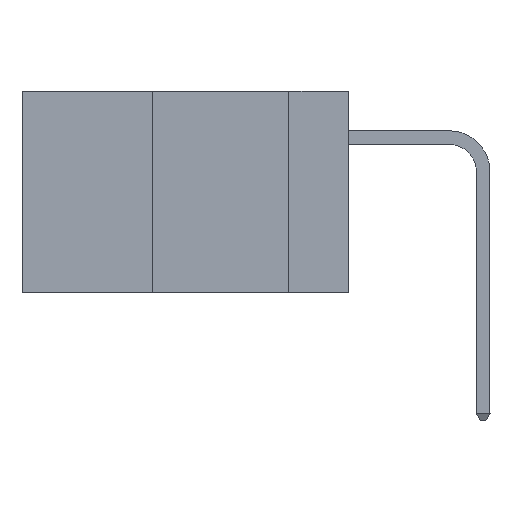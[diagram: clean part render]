
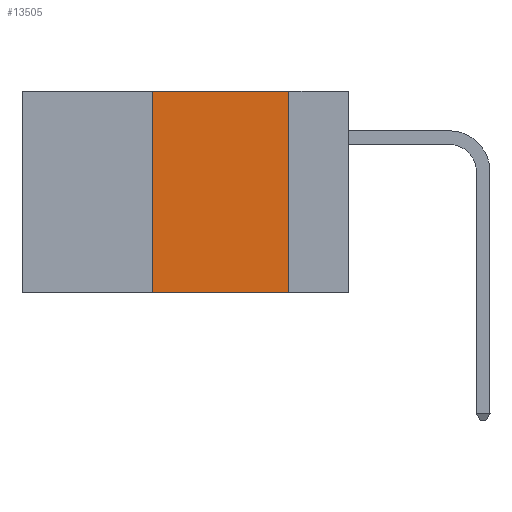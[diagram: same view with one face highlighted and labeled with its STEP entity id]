
A CAD part, left-side view. The second image highlights one B-rep face of the part: STEP entity #13505.
In plain terms, the highlighted planar face has unit normal (-1, 0, 0).
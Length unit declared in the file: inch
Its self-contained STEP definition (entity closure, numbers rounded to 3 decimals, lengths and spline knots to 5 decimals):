
#1385 = EDGE_CURVE ( 'NONE', #3851, #40152, #15248, .T. ) ;
#3851 = VERTEX_POINT ( 'NONE', #22185 ) ;
#4077 = CARTESIAN_POINT ( 'NONE',  ( 0., 0.36, 0. ) ) ;
#4573 = DIRECTION ( 'NONE',  ( 0., 0., -1. ) ) ;
#5315 = CARTESIAN_POINT ( 'NONE',  ( 0., 0.11, 0. ) ) ;
#6970 = VECTOR ( 'NONE', #32015, 39.37008 ) ;
#7897 = CARTESIAN_POINT ( 'NONE',  ( 0., 0.36, 0. ) ) ;
#8837 = CARTESIAN_POINT ( 'NONE',  ( 0., 0.6, 0. ) ) ;
#9611 = LINE ( 'NONE', #26953, #22558 ) ;
#10759 = ORIENTED_EDGE ( 'NONE', *, *, #25323, .T. ) ;
#11926 = EDGE_CURVE ( 'NONE', #40152, #25382, #15953, .T. ) ;
#12947 = DIRECTION ( 'NONE',  ( 0., -1., 0. ) ) ;
#13505 = ADVANCED_FACE ( 'NONE', ( #25249 ), #34825, .F. ) ;
#15248 = LINE ( 'NONE', #7897, #15716 ) ;
#15716 = VECTOR ( 'NONE', #28805, 39.37008 ) ;
#15953 = LINE ( 'NONE', #8837, #27984 ) ;
#17704 = DIRECTION ( 'NONE',  ( 1., 0., 0. ) ) ;
#22185 = CARTESIAN_POINT ( 'NONE',  ( 0., 0.36, -0.37 ) ) ;
#22558 = VECTOR ( 'NONE', #12947, 39.37008 ) ;
#23162 = EDGE_LOOP ( 'NONE', ( #31572, #28137, #36270, #10759 ) ) ;
#25249 = FACE_OUTER_BOUND ( 'NONE', #23162, .T. ) ;
#25323 = EDGE_CURVE ( 'NONE', #3851, #27844, #9611, .T. ) ;
#25382 = VERTEX_POINT ( 'NONE', #40768 ) ;
#26953 = CARTESIAN_POINT ( 'NONE',  ( 0., 0.6, -0.37 ) ) ;
#27844 = VERTEX_POINT ( 'NONE', #35292 ) ;
#27984 = VECTOR ( 'NONE', #39996, 39.37008 ) ;
#28137 = ORIENTED_EDGE ( 'NONE', *, *, #11926, .F. ) ;
#28805 = DIRECTION ( 'NONE',  ( 0., 0., 1. ) ) ;
#31572 = ORIENTED_EDGE ( 'NONE', *, *, #38902, .F. ) ;
#31579 = LINE ( 'NONE', #5315, #6970 ) ;
#31980 = AXIS2_PLACEMENT_3D ( 'NONE', #35272, #17704, #4573 ) ;
#32015 = DIRECTION ( 'NONE',  ( 0., 0., -1. ) ) ;
#34825 = PLANE ( 'NONE',  #31980 ) ;
#35272 = CARTESIAN_POINT ( 'NONE',  ( 0., 0.6, 0. ) ) ;
#35292 = CARTESIAN_POINT ( 'NONE',  ( 0., 0.11, -0.37 ) ) ;
#36270 = ORIENTED_EDGE ( 'NONE', *, *, #1385, .F. ) ;
#38902 = EDGE_CURVE ( 'NONE', #25382, #27844, #31579, .T. ) ;
#39996 = DIRECTION ( 'NONE',  ( 0., -1., 0. ) ) ;
#40152 = VERTEX_POINT ( 'NONE', #4077 ) ;
#40768 = CARTESIAN_POINT ( 'NONE',  ( 0., 0.11, 0. ) ) ;
